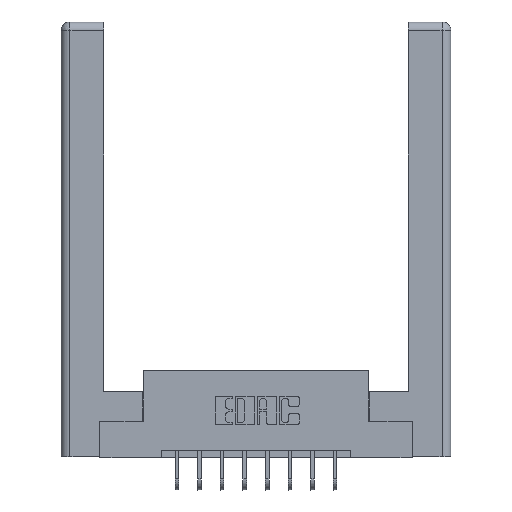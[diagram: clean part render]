
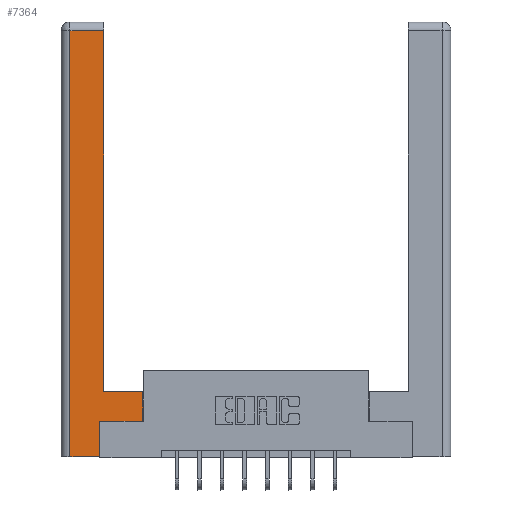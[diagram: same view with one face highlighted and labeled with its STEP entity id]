
A CAD part, top view. The second image highlights one B-rep face of the part: STEP entity #7364.
In plain terms, the highlighted planar face has unit normal (0, 0, 1).
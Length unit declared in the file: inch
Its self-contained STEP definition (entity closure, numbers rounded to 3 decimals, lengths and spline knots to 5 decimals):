
#124 = CARTESIAN_POINT ( 'NONE',  ( 0.265, 0., 0. ) ) ;
#215 = EDGE_CURVE ( 'NONE', #5062, #11185, #2766, .T. ) ;
#787 = CARTESIAN_POINT ( 'NONE',  ( 0.565, 0.245, 0. ) ) ;
#878 = EDGE_CURVE ( 'NONE', #3214, #10129, #5448, .T. ) ;
#1403 = DIRECTION ( 'NONE',  ( 0., -1., 0. ) ) ;
#1418 = VERTEX_POINT ( 'NONE', #5453 ) ;
#1632 = ORIENTED_EDGE ( 'NONE', *, *, #9289, .T. ) ;
#1738 = CARTESIAN_POINT ( 'NONE',  ( 0.295, 0.45, 0. ) ) ;
#1785 = AXIS2_PLACEMENT_3D ( 'NONE', #4142, #5380, #10029 ) ;
#1875 = EDGE_CURVE ( 'NONE', #11185, #3214, #8277, .T. ) ;
#1900 = EDGE_CURVE ( 'NONE', #1418, #5062, #12502, .T. ) ;
#1973 = EDGE_CURVE ( 'NONE', #4637, #10580, #8838, .T. ) ;
#2134 = CARTESIAN_POINT ( 'NONE',  ( 0.565, 0.45, 0. ) ) ;
#2221 = DIRECTION ( 'NONE',  ( 0., 1., 0. ) ) ;
#2313 = VECTOR ( 'NONE', #14300, 39.37008 ) ;
#2416 = ORIENTED_EDGE ( 'NONE', *, *, #1973, .T. ) ;
#2637 = EDGE_CURVE ( 'NONE', #10129, #4637, #13186, .T. ) ;
#2766 = LINE ( 'NONE', #124, #11669 ) ;
#3115 = CARTESIAN_POINT ( 'NONE',  ( 0.265, 0.245, 0. ) ) ;
#3214 = VERTEX_POINT ( 'NONE', #3115 ) ;
#3518 = CARTESIAN_POINT ( 'NONE',  ( 0.565, 0.245, 0. ) ) ;
#3540 = FACE_OUTER_BOUND ( 'NONE', #13554, .T. ) ;
#4142 = CARTESIAN_POINT ( 'NONE',  ( 0., 0., 0. ) ) ;
#4243 = ORIENTED_EDGE ( 'NONE', *, *, #1875, .T. ) ;
#4637 = VERTEX_POINT ( 'NONE', #11619 ) ;
#5062 = VERTEX_POINT ( 'NONE', #13870 ) ;
#5380 = DIRECTION ( 'NONE',  ( 0., 0., -1. ) ) ;
#5448 = LINE ( 'NONE', #787, #2313 ) ;
#5453 = CARTESIAN_POINT ( 'NONE',  ( 0.0615, 2.94, 0. ) ) ;
#5988 = CARTESIAN_POINT ( 'NONE',  ( 0.295, 0.45, 0. ) ) ;
#6309 = VECTOR ( 'NONE', #1403, 39.37008 ) ;
#6587 = CARTESIAN_POINT ( 'NONE',  ( 0.295, 2.94, 0. ) ) ;
#6934 = CARTESIAN_POINT ( 'NONE',  ( 0.0615, 2.94, 0. ) ) ;
#7364 = ADVANCED_FACE ( 'NONE', ( #3540 ), #8750, .F. ) ;
#7401 = VECTOR ( 'NONE', #9637, 39.37008 ) ;
#7734 = VERTEX_POINT ( 'NONE', #6587 ) ;
#7973 = CARTESIAN_POINT ( 'NONE',  ( 0.265, 0.245, 0. ) ) ;
#8172 = DIRECTION ( 'NONE',  ( 1., 0., 0. ) ) ;
#8277 = LINE ( 'NONE', #7973, #14100 ) ;
#8458 = ORIENTED_EDGE ( 'NONE', *, *, #2637, .T. ) ;
#8466 = VECTOR ( 'NONE', #14119, 39.37008 ) ;
#8549 = CARTESIAN_POINT ( 'NONE',  ( 0.295, 3., 0. ) ) ;
#8750 = PLANE ( 'NONE',  #1785 ) ;
#8838 = LINE ( 'NONE', #5988, #8466 ) ;
#9289 = EDGE_CURVE ( 'NONE', #7734, #1418, #14015, .T. ) ;
#9637 = DIRECTION ( 'NONE',  ( 0., 1., 0. ) ) ;
#10029 = DIRECTION ( 'NONE',  ( -1., 0., 0. ) ) ;
#10099 = VECTOR ( 'NONE', #2221, 39.37008 ) ;
#10129 = VERTEX_POINT ( 'NONE', #3518 ) ;
#10133 = ORIENTED_EDGE ( 'NONE', *, *, #878, .T. ) ;
#10580 = VERTEX_POINT ( 'NONE', #1738 ) ;
#10659 = DIRECTION ( 'NONE',  ( -1., 0., 0. ) ) ;
#10731 = ORIENTED_EDGE ( 'NONE', *, *, #11935, .T. ) ;
#11022 = ORIENTED_EDGE ( 'NONE', *, *, #1900, .T. ) ;
#11185 = VERTEX_POINT ( 'NONE', #13466 ) ;
#11619 = CARTESIAN_POINT ( 'NONE',  ( 0.565, 0.45, 0. ) ) ;
#11669 = VECTOR ( 'NONE', #8172, 39.37008 ) ;
#11766 = DIRECTION ( 'NONE',  ( 0., 1., 0. ) ) ;
#11935 = EDGE_CURVE ( 'NONE', #10580, #7734, #11972, .T. ) ;
#11972 = LINE ( 'NONE', #8549, #7401 ) ;
#12502 = LINE ( 'NONE', #13015, #6309 ) ;
#13015 = CARTESIAN_POINT ( 'NONE',  ( 0.0615, 0., 0. ) ) ;
#13186 = LINE ( 'NONE', #2134, #10099 ) ;
#13466 = CARTESIAN_POINT ( 'NONE',  ( 0.265, 0., 0. ) ) ;
#13554 = EDGE_LOOP ( 'NONE', ( #10731, #1632, #11022, #14272, #4243, #10133, #8458, #2416 ) ) ;
#13870 = CARTESIAN_POINT ( 'NONE',  ( 0.0615, 0., 0. ) ) ;
#14015 = LINE ( 'NONE', #6934, #14744 ) ;
#14100 = VECTOR ( 'NONE', #11766, 39.37008 ) ;
#14119 = DIRECTION ( 'NONE',  ( -1., 0., 0. ) ) ;
#14272 = ORIENTED_EDGE ( 'NONE', *, *, #215, .T. ) ;
#14300 = DIRECTION ( 'NONE',  ( 1., 0., 0. ) ) ;
#14744 = VECTOR ( 'NONE', #10659, 39.37008 ) ;
